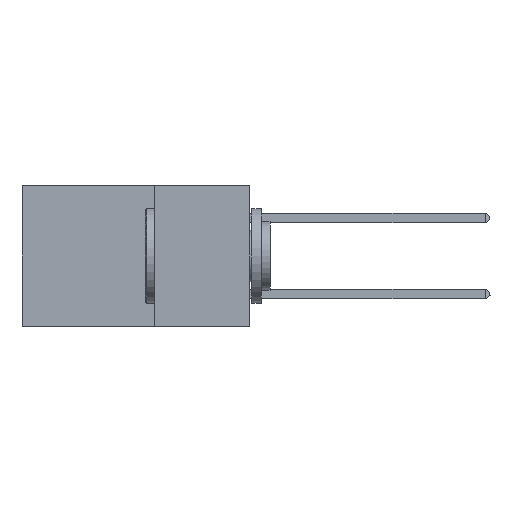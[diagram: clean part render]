
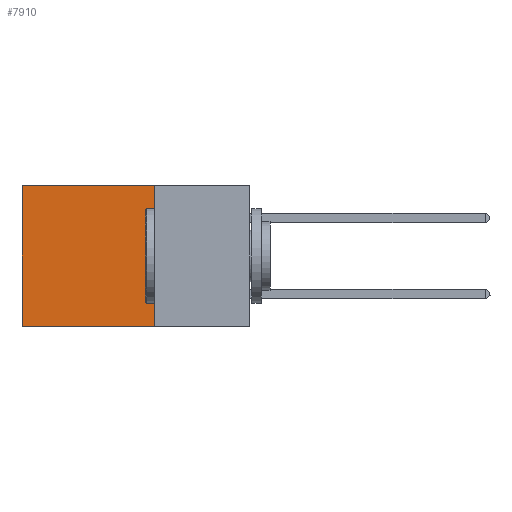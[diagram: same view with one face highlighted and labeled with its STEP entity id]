
A CAD part, left-side view. The second image highlights one B-rep face of the part: STEP entity #7910.
In plain terms, the highlighted planar face has unit normal (-1, 0, 0).
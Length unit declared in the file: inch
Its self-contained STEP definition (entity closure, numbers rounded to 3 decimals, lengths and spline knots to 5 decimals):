
#873 = DIRECTION ( 'NONE',  ( 0., 0., -1. ) ) ;
#1149 = VECTOR ( 'NONE', #7019, 39.37008 ) ;
#1428 = ORIENTED_EDGE ( 'NONE', *, *, #13466, .T. ) ;
#1814 = CARTESIAN_POINT ( 'NONE',  ( 0.2875, 0.25, 0. ) ) ;
#3064 = CARTESIAN_POINT ( 'NONE',  ( 0.2875, 0.25, -0.37 ) ) ;
#3239 = CARTESIAN_POINT ( 'NONE',  ( 0.2875, 0.6, 0. ) ) ;
#3560 = CARTESIAN_POINT ( 'NONE',  ( 0.2875, 0.25, -0.37 ) ) ;
#3597 = EDGE_CURVE ( 'NONE', #15142, #14960, #15706, .T. ) ;
#4602 = VECTOR ( 'NONE', #10131, 39.37008 ) ;
#4810 = CARTESIAN_POINT ( 'NONE',  ( 0.2875, 0.6, -0.37 ) ) ;
#5980 = EDGE_CURVE ( 'NONE', #9026, #15142, #9989, .T. ) ;
#6244 = LINE ( 'NONE', #1814, #1149 ) ;
#7019 = DIRECTION ( 'NONE',  ( 0., 1., 0. ) ) ;
#7149 = VERTEX_POINT ( 'NONE', #3239 ) ;
#7329 = PLANE ( 'NONE',  #16240 ) ;
#7726 = LINE ( 'NONE', #12238, #10528 ) ;
#7910 = ADVANCED_FACE ( 'NONE', ( #10825 ), #7329, .F. ) ;
#8199 = ORIENTED_EDGE ( 'NONE', *, *, #3597, .F. ) ;
#9026 = VERTEX_POINT ( 'NONE', #10404 ) ;
#9781 = VECTOR ( 'NONE', #13801, 39.37008 ) ;
#9962 = CARTESIAN_POINT ( 'NONE',  ( 0.2875, 0.25, 0. ) ) ;
#9967 = ORIENTED_EDGE ( 'NONE', *, *, #5980, .F. ) ;
#9989 = LINE ( 'NONE', #9962, #9781 ) ;
#10131 = DIRECTION ( 'NONE',  ( 0., 1., 0. ) ) ;
#10404 = CARTESIAN_POINT ( 'NONE',  ( 0.2875, 0.25, 0. ) ) ;
#10528 = VECTOR ( 'NONE', #16275, 39.37008 ) ;
#10580 = EDGE_LOOP ( 'NONE', ( #1428, #8199, #9967, #11784 ) ) ;
#10825 = FACE_OUTER_BOUND ( 'NONE', #10580, .T. ) ;
#11784 = ORIENTED_EDGE ( 'NONE', *, *, #15309, .T. ) ;
#12238 = CARTESIAN_POINT ( 'NONE',  ( 0.2875, 0.6, 0. ) ) ;
#12473 = DIRECTION ( 'NONE',  ( 1., 0., 0. ) ) ;
#13466 = EDGE_CURVE ( 'NONE', #7149, #14960, #7726, .T. ) ;
#13801 = DIRECTION ( 'NONE',  ( 0., 0., -1. ) ) ;
#14960 = VERTEX_POINT ( 'NONE', #4810 ) ;
#15142 = VERTEX_POINT ( 'NONE', #3064 ) ;
#15309 = EDGE_CURVE ( 'NONE', #9026, #7149, #6244, .T. ) ;
#15706 = LINE ( 'NONE', #3560, #4602 ) ;
#16240 = AXIS2_PLACEMENT_3D ( 'NONE', #16371, #12473, #873 ) ;
#16275 = DIRECTION ( 'NONE',  ( 0., 0., -1. ) ) ;
#16371 = CARTESIAN_POINT ( 'NONE',  ( 0.2875, 0.25, 0. ) ) ;
